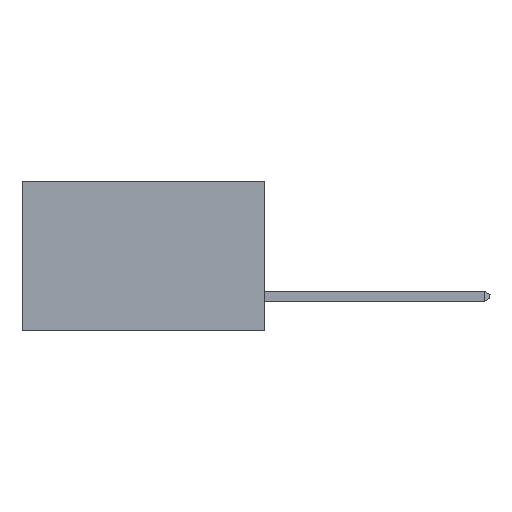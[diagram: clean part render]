
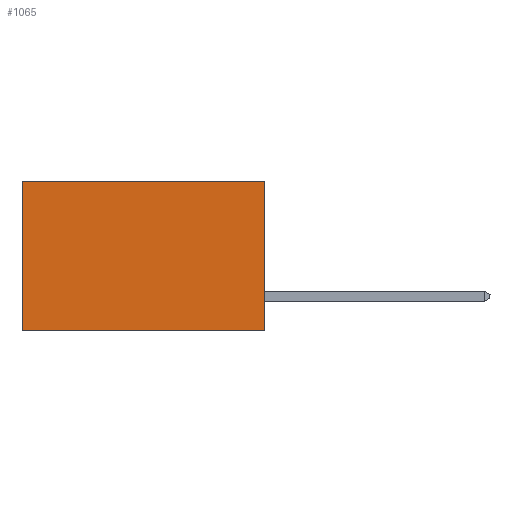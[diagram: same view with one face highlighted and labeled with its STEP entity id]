
A CAD part, left-side view. The second image highlights one B-rep face of the part: STEP entity #1065.
In plain terms, the highlighted planar face has unit normal (-1, 0, 0).
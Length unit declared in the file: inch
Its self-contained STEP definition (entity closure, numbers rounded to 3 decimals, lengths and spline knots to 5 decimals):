
#502 = LINE ( 'NONE', #6476, #8851 ) ;
#816 = CARTESIAN_POINT ( 'NONE',  ( 0.298, 0.6, 0. ) ) ;
#1065 = ADVANCED_FACE ( 'NONE', ( #11263 ), #8429, .F. ) ;
#1225 = ORIENTED_EDGE ( 'NONE', *, *, #10830, .F. ) ;
#2343 = CARTESIAN_POINT ( 'NONE',  ( 0.298, 0., 0. ) ) ;
#2370 = CARTESIAN_POINT ( 'NONE',  ( 0.298, 0.6, -0.37 ) ) ;
#2485 = VECTOR ( 'NONE', #6283, 39.37008 ) ;
#2865 = VERTEX_POINT ( 'NONE', #816 ) ;
#3232 = DIRECTION ( 'NONE',  ( 0., 0., -1. ) ) ;
#3557 = CARTESIAN_POINT ( 'NONE',  ( 0.298, 0., 0. ) ) ;
#4048 = AXIS2_PLACEMENT_3D ( 'NONE', #2343, #11076, #3232 ) ;
#4600 = ORIENTED_EDGE ( 'NONE', *, *, #8311, .F. ) ;
#4866 = LINE ( 'NONE', #10880, #8967 ) ;
#5239 = ORIENTED_EDGE ( 'NONE', *, *, #9612, .T. ) ;
#5528 = EDGE_LOOP ( 'NONE', ( #5239, #1225, #4600, #10014 ) ) ;
#5642 = DIRECTION ( 'NONE',  ( 0., 1., 0. ) ) ;
#6031 = LINE ( 'NONE', #3557, #2485 ) ;
#6283 = DIRECTION ( 'NONE',  ( 0., 1., 0. ) ) ;
#6389 = VECTOR ( 'NONE', #5642, 39.37008 ) ;
#6413 = VERTEX_POINT ( 'NONE', #11303 ) ;
#6476 = CARTESIAN_POINT ( 'NONE',  ( 0.298, 0., 0. ) ) ;
#6500 = CARTESIAN_POINT ( 'NONE',  ( 0.298, 0., 0. ) ) ;
#6919 = EDGE_CURVE ( 'NONE', #9834, #2865, #6031, .T. ) ;
#7191 = LINE ( 'NONE', #9160, #6389 ) ;
#7327 = DIRECTION ( 'NONE',  ( 0., 0., -1. ) ) ;
#7635 = VERTEX_POINT ( 'NONE', #2370 ) ;
#8311 = EDGE_CURVE ( 'NONE', #9834, #6413, #502, .T. ) ;
#8429 = PLANE ( 'NONE',  #4048 ) ;
#8851 = VECTOR ( 'NONE', #7327, 39.37008 ) ;
#8967 = VECTOR ( 'NONE', #9126, 39.37008 ) ;
#9126 = DIRECTION ( 'NONE',  ( 0., 0., -1. ) ) ;
#9160 = CARTESIAN_POINT ( 'NONE',  ( 0.298, 0., -0.37 ) ) ;
#9612 = EDGE_CURVE ( 'NONE', #2865, #7635, #4866, .T. ) ;
#9834 = VERTEX_POINT ( 'NONE', #6500 ) ;
#10014 = ORIENTED_EDGE ( 'NONE', *, *, #6919, .T. ) ;
#10830 = EDGE_CURVE ( 'NONE', #6413, #7635, #7191, .T. ) ;
#10880 = CARTESIAN_POINT ( 'NONE',  ( 0.298, 0.6, 0. ) ) ;
#11076 = DIRECTION ( 'NONE',  ( 1., 0., 0. ) ) ;
#11263 = FACE_OUTER_BOUND ( 'NONE', #5528, .T. ) ;
#11303 = CARTESIAN_POINT ( 'NONE',  ( 0.298, 0., -0.37 ) ) ;
